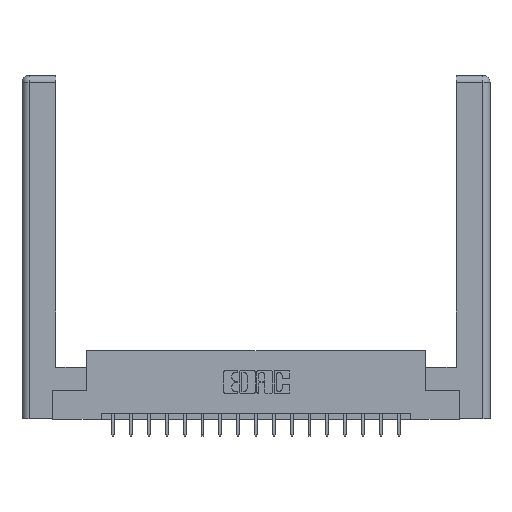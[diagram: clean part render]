
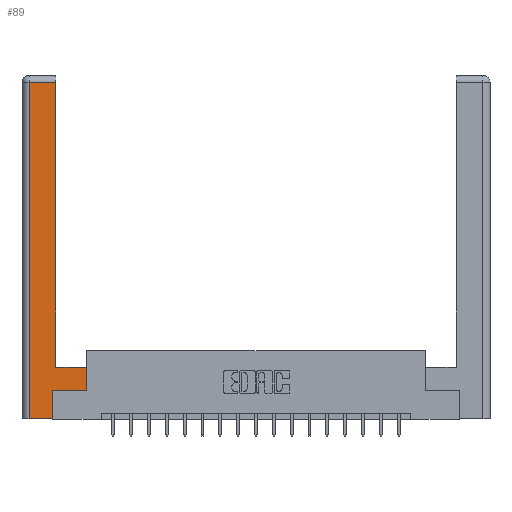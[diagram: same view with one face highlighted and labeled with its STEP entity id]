
A CAD part, top view. The second image highlights one B-rep face of the part: STEP entity #89.
In plain terms, the highlighted planar face has unit normal (0, 0, 1).
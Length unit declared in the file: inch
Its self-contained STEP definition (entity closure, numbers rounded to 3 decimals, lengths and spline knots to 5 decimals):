
#89 = ADVANCED_FACE ( 'NONE', ( #13239 ), #16784, .F. ) ;
#204 = ORIENTED_EDGE ( 'NONE', *, *, #3173, .T. ) ;
#275 = VERTEX_POINT ( 'NONE', #919 ) ;
#863 = EDGE_CURVE ( 'NONE', #4260, #6140, #11548, .T. ) ;
#919 = CARTESIAN_POINT ( 'NONE',  ( 0.295, 2.94, 0. ) ) ;
#924 = ORIENTED_EDGE ( 'NONE', *, *, #863, .T. ) ;
#1165 = CARTESIAN_POINT ( 'NONE',  ( 0.565, 0.45, 0. ) ) ;
#1291 = DIRECTION ( 'NONE',  ( 0., -1., 0. ) ) ;
#1330 = CARTESIAN_POINT ( 'NONE',  ( 0.295, 3., 0. ) ) ;
#1456 = VECTOR ( 'NONE', #13382, 39.37008 ) ;
#1475 = DIRECTION ( 'NONE',  ( 1., 0., 0. ) ) ;
#1631 = CARTESIAN_POINT ( 'NONE',  ( 0.295, 0.45, 0. ) ) ;
#1755 = VECTOR ( 'NONE', #8746, 39.37008 ) ;
#2199 = ORIENTED_EDGE ( 'NONE', *, *, #8036, .T. ) ;
#2524 = DIRECTION ( 'NONE',  ( -1., 0., 0. ) ) ;
#3173 = EDGE_CURVE ( 'NONE', #4575, #11661, #11529, .T. ) ;
#4092 = EDGE_LOOP ( 'NONE', ( #10446, #18289, #7820, #204, #5869, #924, #17869, #2199 ) ) ;
#4125 = VECTOR ( 'NONE', #1291, 39.37008 ) ;
#4260 = VERTEX_POINT ( 'NONE', #8976 ) ;
#4529 = CARTESIAN_POINT ( 'NONE',  ( 0.265, 0.245, 0. ) ) ;
#4552 = CARTESIAN_POINT ( 'NONE',  ( 0.295, 0.45, 0. ) ) ;
#4575 = VERTEX_POINT ( 'NONE', #15916 ) ;
#4592 = DIRECTION ( 'NONE',  ( 0., 1., 0. ) ) ;
#5133 = VECTOR ( 'NONE', #1475, 39.37008 ) ;
#5233 = DIRECTION ( 'NONE',  ( -1., 0., 0. ) ) ;
#5733 = EDGE_CURVE ( 'NONE', #11661, #4260, #9231, .T. ) ;
#5852 = DIRECTION ( 'NONE',  ( -1., 0., 0. ) ) ;
#5869 = ORIENTED_EDGE ( 'NONE', *, *, #5733, .T. ) ;
#6140 = VERTEX_POINT ( 'NONE', #7346 ) ;
#7346 = CARTESIAN_POINT ( 'NONE',  ( 0.565, 0.245, 0. ) ) ;
#7408 = CARTESIAN_POINT ( 'NONE',  ( 0.0615, 2.94, 0. ) ) ;
#7820 = ORIENTED_EDGE ( 'NONE', *, *, #16324, .T. ) ;
#8036 = EDGE_CURVE ( 'NONE', #13578, #10216, #15407, .T. ) ;
#8169 = DIRECTION ( 'NONE',  ( 0., 0., -1. ) ) ;
#8690 = VECTOR ( 'NONE', #5852, 39.37008 ) ;
#8746 = DIRECTION ( 'NONE',  ( 0., 1., 0. ) ) ;
#8976 = CARTESIAN_POINT ( 'NONE',  ( 0.265, 0.245, 0. ) ) ;
#9196 = LINE ( 'NONE', #12718, #9414 ) ;
#9231 = LINE ( 'NONE', #4529, #1456 ) ;
#9233 = VECTOR ( 'NONE', #14628, 39.37008 ) ;
#9414 = VECTOR ( 'NONE', #2524, 39.37008 ) ;
#9520 = LINE ( 'NONE', #1330, #1755 ) ;
#9628 = AXIS2_PLACEMENT_3D ( 'NONE', #12352, #8169, #5233 ) ;
#10216 = VERTEX_POINT ( 'NONE', #4552 ) ;
#10446 = ORIENTED_EDGE ( 'NONE', *, *, #18038, .T. ) ;
#10821 = VECTOR ( 'NONE', #4592, 39.37008 ) ;
#11126 = EDGE_CURVE ( 'NONE', #6140, #13578, #14781, .T. ) ;
#11529 = LINE ( 'NONE', #17490, #9233 ) ;
#11548 = LINE ( 'NONE', #13167, #5133 ) ;
#11661 = VERTEX_POINT ( 'NONE', #11731 ) ;
#11731 = CARTESIAN_POINT ( 'NONE',  ( 0.265, 0., 0. ) ) ;
#12352 = CARTESIAN_POINT ( 'NONE',  ( 0., 0., 0. ) ) ;
#12718 = CARTESIAN_POINT ( 'NONE',  ( 0.0615, 2.94, 0. ) ) ;
#12775 = CARTESIAN_POINT ( 'NONE',  ( 0.0615, 0., 0. ) ) ;
#13167 = CARTESIAN_POINT ( 'NONE',  ( 0.565, 0.245, 0. ) ) ;
#13239 = FACE_OUTER_BOUND ( 'NONE', #4092, .T. ) ;
#13382 = DIRECTION ( 'NONE',  ( 0., 1., 0. ) ) ;
#13578 = VERTEX_POINT ( 'NONE', #1165 ) ;
#14628 = DIRECTION ( 'NONE',  ( 1., 0., 0. ) ) ;
#14661 = CARTESIAN_POINT ( 'NONE',  ( 0.565, 0.45, 0. ) ) ;
#14781 = LINE ( 'NONE', #14661, #10821 ) ;
#15207 = EDGE_CURVE ( 'NONE', #275, #17031, #9196, .T. ) ;
#15407 = LINE ( 'NONE', #1631, #8690 ) ;
#15916 = CARTESIAN_POINT ( 'NONE',  ( 0.0615, 0., 0. ) ) ;
#16324 = EDGE_CURVE ( 'NONE', #17031, #4575, #17737, .T. ) ;
#16784 = PLANE ( 'NONE',  #9628 ) ;
#17031 = VERTEX_POINT ( 'NONE', #7408 ) ;
#17490 = CARTESIAN_POINT ( 'NONE',  ( 0.265, 0., 0. ) ) ;
#17737 = LINE ( 'NONE', #12775, #4125 ) ;
#17869 = ORIENTED_EDGE ( 'NONE', *, *, #11126, .T. ) ;
#18038 = EDGE_CURVE ( 'NONE', #10216, #275, #9520, .T. ) ;
#18289 = ORIENTED_EDGE ( 'NONE', *, *, #15207, .T. ) ;
